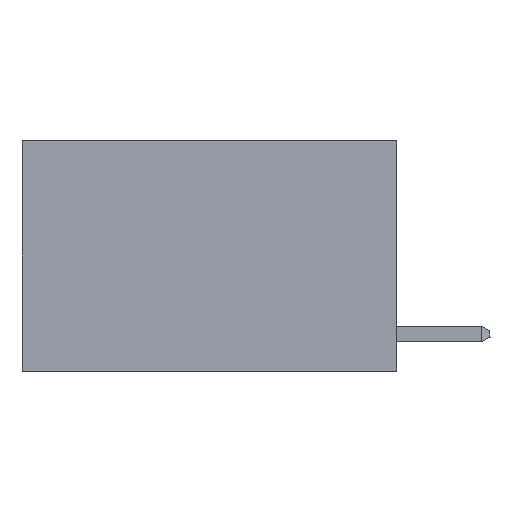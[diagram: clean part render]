
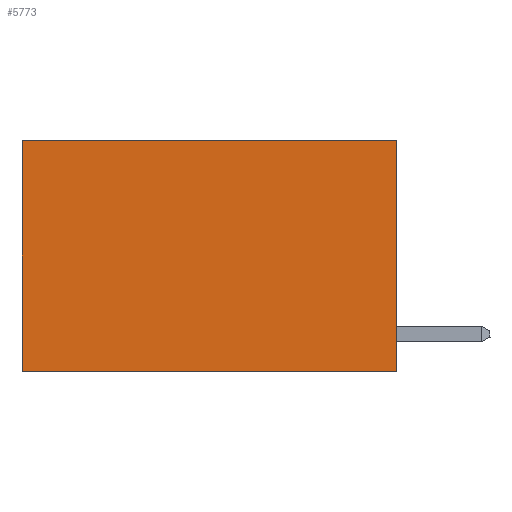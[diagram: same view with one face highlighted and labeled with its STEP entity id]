
A CAD part, left-side view. The second image highlights one B-rep face of the part: STEP entity #5773.
In plain terms, the highlighted planar face has unit normal (-1, 0, 0).
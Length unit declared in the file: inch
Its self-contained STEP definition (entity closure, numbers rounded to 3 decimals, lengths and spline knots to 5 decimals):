
#266 = CARTESIAN_POINT ( 'NONE',  ( 0.2625, 0., -0.37 ) ) ;
#484 = EDGE_LOOP ( 'NONE', ( #9367, #8987, #7097, #8107 ) ) ;
#847 = CARTESIAN_POINT ( 'NONE',  ( 0.2625, 0.6, -0.37 ) ) ;
#913 = AXIS2_PLACEMENT_3D ( 'NONE', #5202, #5110, #5096 ) ;
#2196 = CARTESIAN_POINT ( 'NONE',  ( 0.2625, 0.6, 0. ) ) ;
#2216 = LINE ( 'NONE', #3198, #8232 ) ;
#2342 = DIRECTION ( 'NONE',  ( 0., 1., 0. ) ) ;
#2394 = CARTESIAN_POINT ( 'NONE',  ( 0.2625, 0., -0.37 ) ) ;
#2556 = EDGE_CURVE ( 'NONE', #6308, #9398, #3249, .T. ) ;
#2918 = EDGE_CURVE ( 'NONE', #3066, #9398, #6658, .T. ) ;
#2957 = EDGE_CURVE ( 'NONE', #4322, #3066, #5893, .T. ) ;
#3022 = VECTOR ( 'NONE', #5068, 39.37008 ) ;
#3066 = VERTEX_POINT ( 'NONE', #266 ) ;
#3173 = DIRECTION ( 'NONE',  ( 0., 0., -1. ) ) ;
#3198 = CARTESIAN_POINT ( 'NONE',  ( 0.2625, 0., 0. ) ) ;
#3249 = LINE ( 'NONE', #10123, #3022 ) ;
#3251 = DIRECTION ( 'NONE',  ( 0., 1., 0. ) ) ;
#4322 = VERTEX_POINT ( 'NONE', #8389 ) ;
#4737 = CARTESIAN_POINT ( 'NONE',  ( 0.2625, 0., 0. ) ) ;
#5068 = DIRECTION ( 'NONE',  ( 0., 0., -1. ) ) ;
#5096 = DIRECTION ( 'NONE',  ( 0., 0., -1. ) ) ;
#5110 = DIRECTION ( 'NONE',  ( 1., 0., 0. ) ) ;
#5131 = PLANE ( 'NONE',  #913 ) ;
#5202 = CARTESIAN_POINT ( 'NONE',  ( 0.2625, 0., 0. ) ) ;
#5667 = VECTOR ( 'NONE', #3173, 39.37008 ) ;
#5773 = ADVANCED_FACE ( 'NONE', ( #8635 ), #5131, .F. ) ;
#5893 = LINE ( 'NONE', #4737, #5667 ) ;
#6239 = EDGE_CURVE ( 'NONE', #4322, #6308, #2216, .T. ) ;
#6308 = VERTEX_POINT ( 'NONE', #2196 ) ;
#6658 = LINE ( 'NONE', #2394, #10149 ) ;
#7097 = ORIENTED_EDGE ( 'NONE', *, *, #2957, .F. ) ;
#8107 = ORIENTED_EDGE ( 'NONE', *, *, #6239, .T. ) ;
#8232 = VECTOR ( 'NONE', #3251, 39.37008 ) ;
#8389 = CARTESIAN_POINT ( 'NONE',  ( 0.2625, 0., 0. ) ) ;
#8635 = FACE_OUTER_BOUND ( 'NONE', #484, .T. ) ;
#8987 = ORIENTED_EDGE ( 'NONE', *, *, #2918, .F. ) ;
#9367 = ORIENTED_EDGE ( 'NONE', *, *, #2556, .T. ) ;
#9398 = VERTEX_POINT ( 'NONE', #847 ) ;
#10123 = CARTESIAN_POINT ( 'NONE',  ( 0.2625, 0.6, 0. ) ) ;
#10149 = VECTOR ( 'NONE', #2342, 39.37008 ) ;
